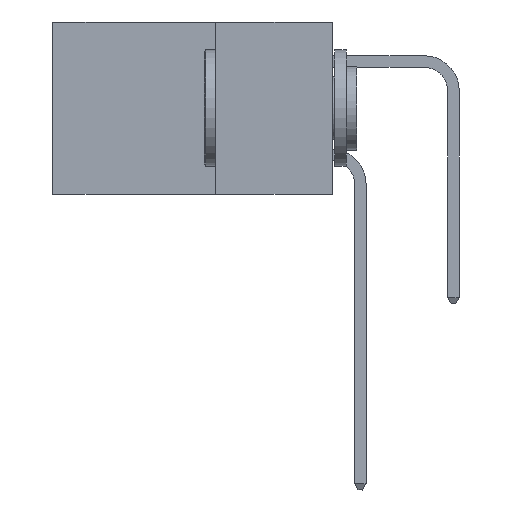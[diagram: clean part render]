
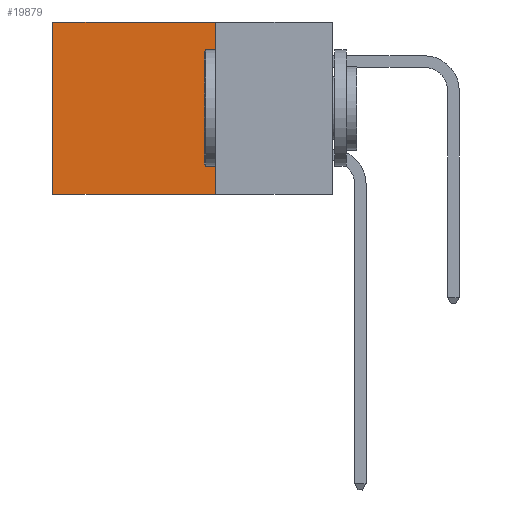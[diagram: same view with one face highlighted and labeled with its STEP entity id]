
A CAD part, left-side view. The second image highlights one B-rep face of the part: STEP entity #19879.
In plain terms, the highlighted planar face has unit normal (-1, 0, 0).
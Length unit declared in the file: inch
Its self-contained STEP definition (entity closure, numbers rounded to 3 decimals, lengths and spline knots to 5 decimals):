
#199 = DIRECTION ( 'NONE',  ( 0., 1., 0. ) ) ;
#830 = EDGE_CURVE ( 'NONE', #14146, #1172, #21453, .T. ) ;
#1053 = EDGE_CURVE ( 'NONE', #18241, #21968, #22977, .T. ) ;
#1172 = VERTEX_POINT ( 'NONE', #17299 ) ;
#1650 = ORIENTED_EDGE ( 'NONE', *, *, #14505, .T. ) ;
#2366 = VECTOR ( 'NONE', #5754, 39.37008 ) ;
#2816 = CARTESIAN_POINT ( 'NONE',  ( 0.2615, 0.25, 0. ) ) ;
#2939 = CARTESIAN_POINT ( 'NONE',  ( 0.2615, 0.25, -0.37 ) ) ;
#3516 = EDGE_CURVE ( 'NONE', #14146, #18241, #5932, .T. ) ;
#5505 = CARTESIAN_POINT ( 'NONE',  ( 0.2615, 0.25, 0. ) ) ;
#5754 = DIRECTION ( 'NONE',  ( 0., 0., -1. ) ) ;
#5918 = ORIENTED_EDGE ( 'NONE', *, *, #830, .T. ) ;
#5932 = LINE ( 'NONE', #22484, #11529 ) ;
#6788 = ORIENTED_EDGE ( 'NONE', *, *, #1053, .F. ) ;
#6871 = VECTOR ( 'NONE', #199, 39.37008 ) ;
#7522 = CARTESIAN_POINT ( 'NONE',  ( 0.2615, 0.6, -0.37 ) ) ;
#8197 = CARTESIAN_POINT ( 'NONE',  ( 0.2615, 0.6, -0.37 ) ) ;
#8525 = AXIS2_PLACEMENT_3D ( 'NONE', #2939, #19488, #17600 ) ;
#9971 = DIRECTION ( 'NONE',  ( 0., 1., 0. ) ) ;
#11171 = VECTOR ( 'NONE', #9971, 39.37008 ) ;
#11529 = VECTOR ( 'NONE', #13135, 39.37008 ) ;
#11758 = CARTESIAN_POINT ( 'NONE',  ( 0.2615, 0.25, -0.37 ) ) ;
#12279 = PLANE ( 'NONE',  #8525 ) ;
#13135 = DIRECTION ( 'NONE',  ( 0., 0., -1. ) ) ;
#13811 = FACE_OUTER_BOUND ( 'NONE', #17697, .T. ) ;
#14146 = VERTEX_POINT ( 'NONE', #2816 ) ;
#14505 = EDGE_CURVE ( 'NONE', #1172, #21968, #16737, .T. ) ;
#15266 = CARTESIAN_POINT ( 'NONE',  ( 0.2615, 0.25, -0.37 ) ) ;
#16683 = ORIENTED_EDGE ( 'NONE', *, *, #3516, .F. ) ;
#16737 = LINE ( 'NONE', #7522, #2366 ) ;
#17299 = CARTESIAN_POINT ( 'NONE',  ( 0.2615, 0.6, 0. ) ) ;
#17600 = DIRECTION ( 'NONE',  ( 0., 0., -1. ) ) ;
#17697 = EDGE_LOOP ( 'NONE', ( #1650, #6788, #16683, #5918 ) ) ;
#18241 = VERTEX_POINT ( 'NONE', #15266 ) ;
#19488 = DIRECTION ( 'NONE',  ( 1., 0., 0. ) ) ;
#19879 = ADVANCED_FACE ( 'NONE', ( #13811 ), #12279, .F. ) ;
#21453 = LINE ( 'NONE', #5505, #6871 ) ;
#21968 = VERTEX_POINT ( 'NONE', #8197 ) ;
#22484 = CARTESIAN_POINT ( 'NONE',  ( 0.2615, 0.25, -0.37 ) ) ;
#22977 = LINE ( 'NONE', #11758, #11171 ) ;
